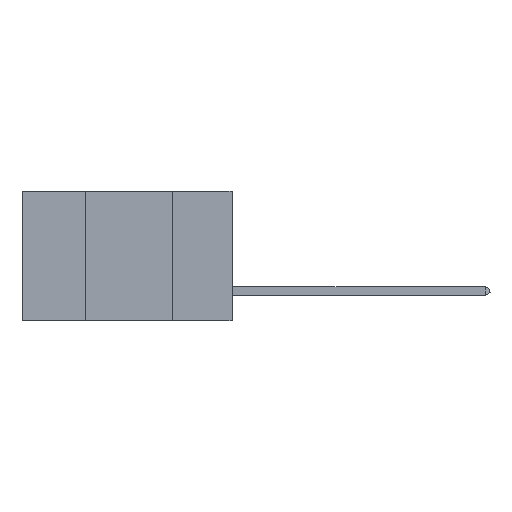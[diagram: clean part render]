
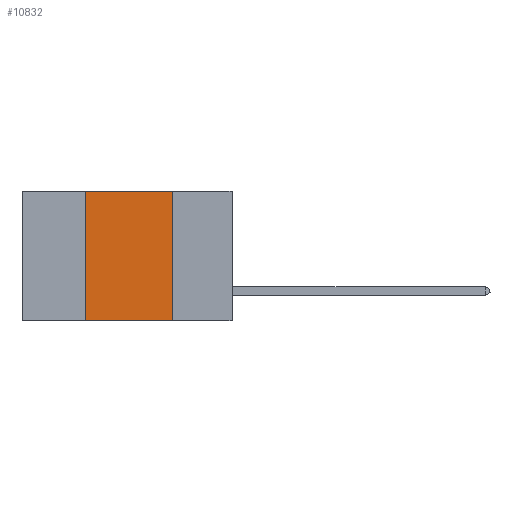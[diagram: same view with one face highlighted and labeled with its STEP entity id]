
A CAD part, left-side view. The second image highlights one B-rep face of the part: STEP entity #10832.
In plain terms, the highlighted planar face has unit normal (-1, 0, 0).
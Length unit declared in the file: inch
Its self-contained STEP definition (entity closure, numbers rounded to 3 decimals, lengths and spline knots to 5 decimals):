
#53 = AXIS2_PLACEMENT_3D ( 'NONE', #11191, #5506, #5549 ) ;
#580 = PLANE ( 'NONE',  #53 ) ;
#931 = EDGE_LOOP ( 'NONE', ( #6681, #10600, #9219, #1663 ) ) ;
#993 = DIRECTION ( 'NONE',  ( 0., 0., 1. ) ) ;
#1025 = VECTOR ( 'NONE', #993, 39.37008 ) ;
#1636 = EDGE_CURVE ( 'NONE', #10285, #2317, #11515, .T. ) ;
#1663 = ORIENTED_EDGE ( 'NONE', *, *, #1636, .T. ) ;
#2115 = VECTOR ( 'NONE', #4667, 39.37008 ) ;
#2317 = VERTEX_POINT ( 'NONE', #6436 ) ;
#2617 = FACE_OUTER_BOUND ( 'NONE', #931, .T. ) ;
#2834 = VERTEX_POINT ( 'NONE', #9941 ) ;
#2883 = LINE ( 'NONE', #5602, #2115 ) ;
#2944 = CARTESIAN_POINT ( 'NONE',  ( 0., 0.42, 0. ) ) ;
#3172 = VECTOR ( 'NONE', #10140, 39.37008 ) ;
#3880 = CARTESIAN_POINT ( 'NONE',  ( 0., 0.6, 0. ) ) ;
#3904 = LINE ( 'NONE', #3880, #4187 ) ;
#4124 = EDGE_CURVE ( 'NONE', #9958, #2834, #3904, .T. ) ;
#4187 = VECTOR ( 'NONE', #11531, 39.37008 ) ;
#4399 = CARTESIAN_POINT ( 'NONE',  ( 0., 0.42, 0. ) ) ;
#4667 = DIRECTION ( 'NONE',  ( 0., 0., -1. ) ) ;
#5506 = DIRECTION ( 'NONE',  ( 1., 0., 0. ) ) ;
#5549 = DIRECTION ( 'NONE',  ( 0., 0., -1. ) ) ;
#5602 = CARTESIAN_POINT ( 'NONE',  ( 0., 0.17, 0. ) ) ;
#6436 = CARTESIAN_POINT ( 'NONE',  ( 0., 0.17, -0.37 ) ) ;
#6681 = ORIENTED_EDGE ( 'NONE', *, *, #11268, .F. ) ;
#7259 = CARTESIAN_POINT ( 'NONE',  ( 0., 0.6, -0.37 ) ) ;
#8352 = EDGE_CURVE ( 'NONE', #10285, #9958, #10187, .T. ) ;
#8995 = CARTESIAN_POINT ( 'NONE',  ( 0., 0.42, -0.37 ) ) ;
#9219 = ORIENTED_EDGE ( 'NONE', *, *, #8352, .F. ) ;
#9941 = CARTESIAN_POINT ( 'NONE',  ( 0., 0.17, 0. ) ) ;
#9958 = VERTEX_POINT ( 'NONE', #4399 ) ;
#10140 = DIRECTION ( 'NONE',  ( 0., -1., 0. ) ) ;
#10187 = LINE ( 'NONE', #2944, #1025 ) ;
#10285 = VERTEX_POINT ( 'NONE', #8995 ) ;
#10600 = ORIENTED_EDGE ( 'NONE', *, *, #4124, .F. ) ;
#10832 = ADVANCED_FACE ( 'NONE', ( #2617 ), #580, .F. ) ;
#11191 = CARTESIAN_POINT ( 'NONE',  ( 0., 0.6, 0. ) ) ;
#11268 = EDGE_CURVE ( 'NONE', #2834, #2317, #2883, .T. ) ;
#11515 = LINE ( 'NONE', #7259, #3172 ) ;
#11531 = DIRECTION ( 'NONE',  ( 0., -1., 0. ) ) ;
